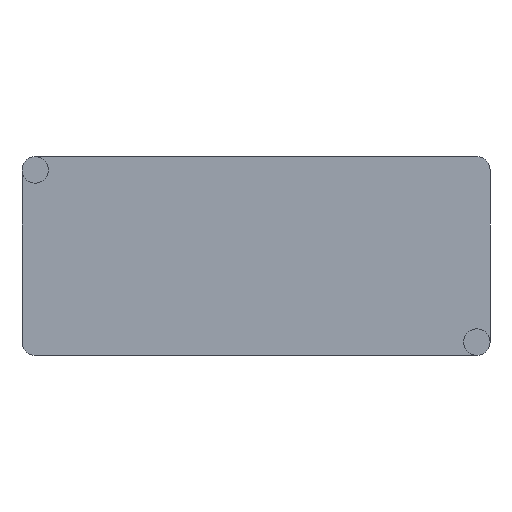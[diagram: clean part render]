
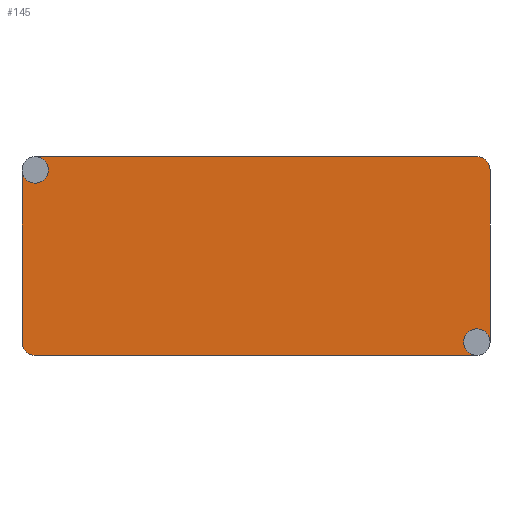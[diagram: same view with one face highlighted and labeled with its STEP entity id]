
A CAD part, top view. The second image highlights one B-rep face of the part: STEP entity #145.
In plain terms, the highlighted planar face has unit normal (0, 0, 1).
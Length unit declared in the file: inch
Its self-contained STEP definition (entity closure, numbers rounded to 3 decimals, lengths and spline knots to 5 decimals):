
#1 = CARTESIAN_POINT ( 'NONE',  ( 0.98425, 0.38386, -0.17717 ) ) ;
#3 = CARTESIAN_POINT ( 'NONE',  ( -0.9252, 0.38386, -0.17717 ) ) ;
#16 = ORIENTED_EDGE ( 'NONE', *, *, #404, .T. ) ;
#33 = VECTOR ( 'NONE', #126, 39.37008 ) ;
#36 = ORIENTED_EDGE ( 'NONE', *, *, #403, .T. ) ;
#38 = VERTEX_POINT ( 'NONE', #116 ) ;
#39 = DIRECTION ( 'NONE',  ( 1., 0., 0. ) ) ;
#43 = CARTESIAN_POINT ( 'NONE',  ( 0.98425, -0.38386, -0.17717 ) ) ;
#48 = PLANE ( 'NONE',  #350 ) ;
#51 = ORIENTED_EDGE ( 'NONE', *, *, #399, .T. ) ;
#55 = DIRECTION ( 'NONE',  ( 0., 0., 1. ) ) ;
#61 = VERTEX_POINT ( 'NONE', #183 ) ;
#63 = EDGE_LOOP ( 'NONE', ( #208, #475, #79, #248, #154, #479, #16, #36, #51, #379 ) ) ;
#68 = VERTEX_POINT ( 'NONE', #227 ) ;
#72 = VECTOR ( 'NONE', #217, 39.37008 ) ;
#73 = CARTESIAN_POINT ( 'NONE',  ( 0.98425, 0.44291, -0.17717 ) ) ;
#79 = ORIENTED_EDGE ( 'NONE', *, *, #421, .F. ) ;
#81 = DIRECTION ( 'NONE',  ( 1., 0., 0. ) ) ;
#113 = DIRECTION ( 'NONE',  ( 0., 0., 1. ) ) ;
#116 = CARTESIAN_POINT ( 'NONE',  ( 0.98425, -0.44291, -0.17717 ) ) ;
#123 = VERTEX_POINT ( 'NONE', #323 ) ;
#126 = DIRECTION ( 'NONE',  ( 0., -1., 0. ) ) ;
#144 = CIRCLE ( 'NONE', #266, 0.05906 ) ;
#145 = ADVANCED_FACE ( 'NONE', ( #330 ), #48, .F. ) ;
#147 = LINE ( 'NONE', #198, #33 ) ;
#151 = DIRECTION ( 'NONE',  ( 0., 0., -1. ) ) ;
#153 = CARTESIAN_POINT ( 'NONE',  ( -0.98425, 0.38386, -0.17717 ) ) ;
#154 = ORIENTED_EDGE ( 'NONE', *, *, #427, .F. ) ;
#165 = CIRCLE ( 'NONE', #288, 0.05906 ) ;
#166 = VERTEX_POINT ( 'NONE', #233 ) ;
#177 = CARTESIAN_POINT ( 'NONE',  ( 0., -0.44291, -0.17717 ) ) ;
#182 = DIRECTION ( 'NONE',  ( 0., 0., -1. ) ) ;
#183 = CARTESIAN_POINT ( 'NONE',  ( -0.98425, -0.44291, -0.17717 ) ) ;
#190 = DIRECTION ( 'NONE',  ( 1., 0., 0. ) ) ;
#198 = CARTESIAN_POINT ( 'NONE',  ( -1.04331, 0., -0.17717 ) ) ;
#206 = CIRCLE ( 'NONE', #251, 0.05906 ) ;
#208 = ORIENTED_EDGE ( 'NONE', *, *, #440, .F. ) ;
#211 = CARTESIAN_POINT ( 'NONE',  ( -1.04331, -0.38386, -0.17717 ) ) ;
#217 = DIRECTION ( 'NONE',  ( 0., 1., 0. ) ) ;
#227 = CARTESIAN_POINT ( 'NONE',  ( 0.9252, -0.38386, -0.17717 ) ) ;
#233 = CARTESIAN_POINT ( 'NONE',  ( -0.98425, 0.44291, -0.17717 ) ) ;
#239 = CIRCLE ( 'NONE', #257, 0.05906 ) ;
#246 = VERTEX_POINT ( 'NONE', #423 ) ;
#248 = ORIENTED_EDGE ( 'NONE', *, *, #407, .T. ) ;
#251 = AXIS2_PLACEMENT_3D ( 'NONE', #283, #55, #329 ) ;
#254 = AXIS2_PLACEMENT_3D ( 'NONE', #153, #462, #190 ) ;
#257 = AXIS2_PLACEMENT_3D ( 'NONE', #374, #113, #419 ) ;
#264 = DIRECTION ( 'NONE',  ( 0., 0., 1. ) ) ;
#266 = AXIS2_PLACEMENT_3D ( 'NONE', #43, #318, #81 ) ;
#267 = AXIS2_PLACEMENT_3D ( 'NONE', #453, #182, #486 ) ;
#281 = LINE ( 'NONE', #447, #72 ) ;
#283 = CARTESIAN_POINT ( 'NONE',  ( -0.98425, 0.38386, -0.17717 ) ) ;
#288 = AXIS2_PLACEMENT_3D ( 'NONE', #1, #264, #39 ) ;
#294 = VECTOR ( 'NONE', #483, 39.37008 ) ;
#318 = DIRECTION ( 'NONE',  ( 0., 0., 1. ) ) ;
#323 = CARTESIAN_POINT ( 'NONE',  ( -1.04331, 0.38386, -0.17717 ) ) ;
#329 = DIRECTION ( 'NONE',  ( 1., 0., 0. ) ) ;
#330 = FACE_OUTER_BOUND ( 'NONE', #63, .T. ) ;
#349 = CIRCLE ( 'NONE', #254, 0.05906 ) ;
#350 = AXIS2_PLACEMENT_3D ( 'NONE', #375, #151, #461 ) ;
#360 = DIRECTION ( 'NONE',  ( -1., 0., 0. ) ) ;
#369 = EDGE_CURVE ( 'NONE', #123, #386, #147, .T. ) ;
#374 = CARTESIAN_POINT ( 'NONE',  ( 0.98425, -0.38386, -0.17717 ) ) ;
#375 = CARTESIAN_POINT ( 'NONE',  ( 0., 0., -0.17717 ) ) ;
#379 = ORIENTED_EDGE ( 'NONE', *, *, #473, .F. ) ;
#386 = VERTEX_POINT ( 'NONE', #211 ) ;
#399 = EDGE_CURVE ( 'NONE', #401, #166, #505, .T. ) ;
#401 = VERTEX_POINT ( 'NONE', #73 ) ;
#402 = VECTOR ( 'NONE', #360, 39.37008 ) ;
#403 = EDGE_CURVE ( 'NONE', #430, #401, #165, .T. ) ;
#404 = EDGE_CURVE ( 'NONE', #246, #430, #281, .T. ) ;
#407 = EDGE_CURVE ( 'NONE', #61, #38, #496, .T. ) ;
#411 = CARTESIAN_POINT ( 'NONE',  ( 1.04331, 0.38386, -0.17717 ) ) ;
#418 = VERTEX_POINT ( 'NONE', #3 ) ;
#419 = DIRECTION ( 'NONE',  ( 1., 0., 0. ) ) ;
#421 = EDGE_CURVE ( 'NONE', #61, #386, #481, .T. ) ;
#423 = CARTESIAN_POINT ( 'NONE',  ( 1.04331, -0.38386, -0.17717 ) ) ;
#427 = EDGE_CURVE ( 'NONE', #68, #38, #144, .T. ) ;
#430 = VERTEX_POINT ( 'NONE', #411 ) ;
#432 = EDGE_CURVE ( 'NONE', #246, #68, #239, .T. ) ;
#440 = EDGE_CURVE ( 'NONE', #123, #418, #349, .T. ) ;
#447 = CARTESIAN_POINT ( 'NONE',  ( 1.04331, 0., -0.17717 ) ) ;
#453 = CARTESIAN_POINT ( 'NONE',  ( -0.98425, -0.38386, -0.17717 ) ) ;
#461 = DIRECTION ( 'NONE',  ( 1., 0., 0. ) ) ;
#462 = DIRECTION ( 'NONE',  ( 0., 0., 1. ) ) ;
#473 = EDGE_CURVE ( 'NONE', #418, #166, #206, .T. ) ;
#475 = ORIENTED_EDGE ( 'NONE', *, *, #369, .T. ) ;
#479 = ORIENTED_EDGE ( 'NONE', *, *, #432, .F. ) ;
#481 = CIRCLE ( 'NONE', #267, 0.05906 ) ;
#483 = DIRECTION ( 'NONE',  ( 1., 0., 0. ) ) ;
#486 = DIRECTION ( 'NONE',  ( 1., 0., 0. ) ) ;
#496 = LINE ( 'NONE', #177, #294 ) ;
#505 = LINE ( 'NONE', #511, #402 ) ;
#511 = CARTESIAN_POINT ( 'NONE',  ( 0., 0.44291, -0.17717 ) ) ;
